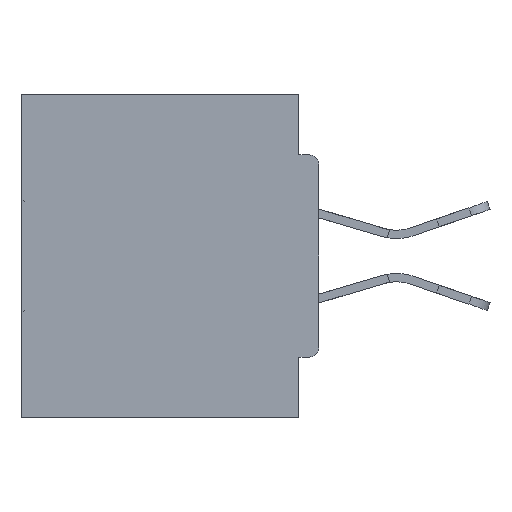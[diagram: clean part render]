
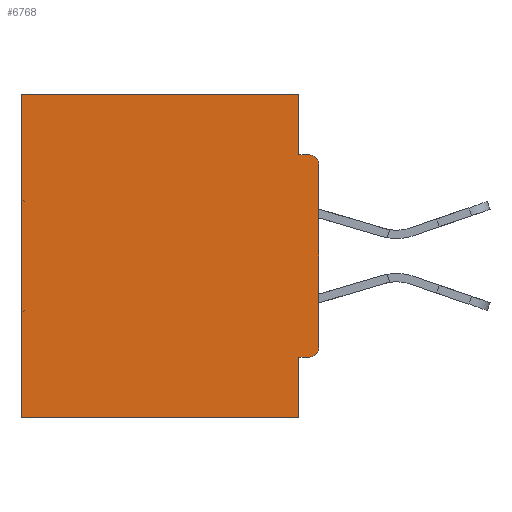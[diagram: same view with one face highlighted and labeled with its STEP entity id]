
A CAD part, left-side view. The second image highlights one B-rep face of the part: STEP entity #6768.
In plain terms, the highlighted planar face has unit normal (-1, 0, 0).
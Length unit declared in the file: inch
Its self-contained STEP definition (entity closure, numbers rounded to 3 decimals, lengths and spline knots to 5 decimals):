
#62 = ORIENTED_EDGE ( 'NONE', *, *, #31509, .F. ) ;
#794 = VERTEX_POINT ( 'NONE', #36047 ) ;
#926 = VECTOR ( 'NONE', #1300, 39.37008 ) ;
#1300 = DIRECTION ( 'NONE',  ( 0., 1., 0. ) ) ;
#1567 = CARTESIAN_POINT ( 'NONE',  ( 0.298, 0.031, 0. ) ) ;
#2746 = CARTESIAN_POINT ( 'NONE',  ( 0.298, 0., -0.4065 ) ) ;
#2751 = ORIENTED_EDGE ( 'NONE', *, *, #35384, .F. ) ;
#5002 = VECTOR ( 'NONE', #16791, 39.37008 ) ;
#5671 = EDGE_CURVE ( 'NONE', #35676, #30336, #21587, .T. ) ;
#5812 = EDGE_CURVE ( 'NONE', #794, #27218, #32672, .T. ) ;
#5937 = ORIENTED_EDGE ( 'NONE', *, *, #7965, .F. ) ;
#6116 = CARTESIAN_POINT ( 'NONE',  ( 0.298, 0.46, 0. ) ) ;
#6743 = DIRECTION ( 'NONE',  ( 0., 0., -1. ) ) ;
#6768 = ADVANCED_FACE ( 'NONE', ( #29023 ), #19098, .F. ) ;
#7354 = CARTESIAN_POINT ( 'NONE',  ( 0.298, 0.46, 0. ) ) ;
#7462 = EDGE_CURVE ( 'NONE', #38261, #15851, #22695, .T. ) ;
#7965 = EDGE_CURVE ( 'NONE', #15851, #39488, #16873, .T. ) ;
#7985 = EDGE_CURVE ( 'NONE', #38261, #21097, #32724, .T. ) ;
#8307 = CARTESIAN_POINT ( 'NONE',  ( 0.298, 0., 0. ) ) ;
#8450 = AXIS2_PLACEMENT_3D ( 'NONE', #27427, #27571, #27730 ) ;
#8752 = ORIENTED_EDGE ( 'NONE', *, *, #7462, .F. ) ;
#8756 = ORIENTED_EDGE ( 'NONE', *, *, #10908, .T. ) ;
#8794 = VECTOR ( 'NONE', #23334, 39.37008 ) ;
#9895 = CARTESIAN_POINT ( 'NONE',  ( 0.298, 0., -0.5 ) ) ;
#10908 = EDGE_CURVE ( 'NONE', #33389, #27218, #39284, .T. ) ;
#10940 = CARTESIAN_POINT ( 'NONE',  ( 0.298, 0.015, -0.4065 ) ) ;
#11133 = CARTESIAN_POINT ( 'NONE',  ( 0.298, 0., 0. ) ) ;
#11499 = ORIENTED_EDGE ( 'NONE', *, *, #35125, .F. ) ;
#12402 = DIRECTION ( 'NONE',  ( 0., -1., 0. ) ) ;
#13107 = CARTESIAN_POINT ( 'NONE',  ( 0.298, 0., -0.3915 ) ) ;
#13188 = DIRECTION ( 'NONE',  ( 0., 1., 0. ) ) ;
#14216 = CARTESIAN_POINT ( 'NONE',  ( 0.298, 0.015, -0.3915 ) ) ;
#15851 = VERTEX_POINT ( 'NONE', #24425 ) ;
#16791 = DIRECTION ( 'NONE',  ( 0., 0., -1. ) ) ;
#16873 = LINE ( 'NONE', #17031, #41701 ) ;
#17031 = CARTESIAN_POINT ( 'NONE',  ( 0.298, 0.031, -0.5 ) ) ;
#18262 = DIRECTION ( 'NONE',  ( 0., 1., 0. ) ) ;
#18898 = VECTOR ( 'NONE', #12402, 39.37008 ) ;
#19098 = PLANE ( 'NONE',  #39483 ) ;
#19381 = CARTESIAN_POINT ( 'NONE',  ( 0.298, 0., 0. ) ) ;
#20803 = ORIENTED_EDGE ( 'NONE', *, *, #5671, .T. ) ;
#21097 = VERTEX_POINT ( 'NONE', #13107 ) ;
#21587 = LINE ( 'NONE', #6116, #8794 ) ;
#22084 = EDGE_CURVE ( 'NONE', #43184, #35676, #33359, .T. ) ;
#22695 = LINE ( 'NONE', #2746, #29596 ) ;
#23334 = DIRECTION ( 'NONE',  ( 0., 0., -1. ) ) ;
#23855 = CARTESIAN_POINT ( 'NONE',  ( 0.298, 0.031, -0.5 ) ) ;
#24382 = LINE ( 'NONE', #11133, #39679 ) ;
#24425 = CARTESIAN_POINT ( 'NONE',  ( 0.298, 0.031, -0.4065 ) ) ;
#25900 = ORIENTED_EDGE ( 'NONE', *, *, #7985, .T. ) ;
#26260 = EDGE_LOOP ( 'NONE', ( #8756, #35823, #62, #38608, #20803, #2751, #5937, #8752, #25900, #11499 ) ) ;
#26983 = VECTOR ( 'NONE', #13188, 39.37008 ) ;
#27023 = DIRECTION ( 'NONE',  ( -1., 0., 0. ) ) ;
#27218 = VERTEX_POINT ( 'NONE', #32149 ) ;
#27427 = CARTESIAN_POINT ( 'NONE',  ( 0.298, 0.015, -0.1085 ) ) ;
#27571 = DIRECTION ( 'NONE',  ( -1., 0., 0. ) ) ;
#27697 = DIRECTION ( 'NONE',  ( 0., 0., -1. ) ) ;
#27730 = DIRECTION ( 'NONE',  ( 0., 0., -1. ) ) ;
#29023 = FACE_OUTER_BOUND ( 'NONE', #26260, .T. ) ;
#29252 = CARTESIAN_POINT ( 'NONE',  ( 0.298, 0., -0.0935 ) ) ;
#29596 = VECTOR ( 'NONE', #18262, 39.37008 ) ;
#30129 = CARTESIAN_POINT ( 'NONE',  ( 0.298, 0.46, -0.5 ) ) ;
#30336 = VERTEX_POINT ( 'NONE', #30129 ) ;
#31509 = EDGE_CURVE ( 'NONE', #43184, #794, #40510, .T. ) ;
#32149 = CARTESIAN_POINT ( 'NONE',  ( 0.298, 0.015, -0.0935 ) ) ;
#32672 = LINE ( 'NONE', #29252, #18898 ) ;
#32724 = CIRCLE ( 'NONE', #40408, 0.015 ) ;
#33359 = LINE ( 'NONE', #8307, #926 ) ;
#33389 = VERTEX_POINT ( 'NONE', #33684 ) ;
#33684 = CARTESIAN_POINT ( 'NONE',  ( 0.298, 0., -0.1085 ) ) ;
#35125 = EDGE_CURVE ( 'NONE', #33389, #21097, #24382, .T. ) ;
#35384 = EDGE_CURVE ( 'NONE', #39488, #30336, #36001, .T. ) ;
#35676 = VERTEX_POINT ( 'NONE', #7354 ) ;
#35823 = ORIENTED_EDGE ( 'NONE', *, *, #5812, .F. ) ;
#36001 = LINE ( 'NONE', #9895, #26983 ) ;
#36047 = CARTESIAN_POINT ( 'NONE',  ( 0.298, 0.031, -0.0935 ) ) ;
#38261 = VERTEX_POINT ( 'NONE', #10940 ) ;
#38608 = ORIENTED_EDGE ( 'NONE', *, *, #22084, .T. ) ;
#39284 = CIRCLE ( 'NONE', #8450, 0.015 ) ;
#39483 = AXIS2_PLACEMENT_3D ( 'NONE', #19381, #40666, #43477 ) ;
#39488 = VERTEX_POINT ( 'NONE', #43769 ) ;
#39679 = VECTOR ( 'NONE', #27697, 39.37008 ) ;
#40408 = AXIS2_PLACEMENT_3D ( 'NONE', #14216, #27023, #6743 ) ;
#40510 = LINE ( 'NONE', #23855, #5002 ) ;
#40666 = DIRECTION ( 'NONE',  ( 1., 0., 0. ) ) ;
#40794 = DIRECTION ( 'NONE',  ( 0., 0., -1. ) ) ;
#41701 = VECTOR ( 'NONE', #40794, 39.37008 ) ;
#43184 = VERTEX_POINT ( 'NONE', #1567 ) ;
#43477 = DIRECTION ( 'NONE',  ( 0., 0., -1. ) ) ;
#43769 = CARTESIAN_POINT ( 'NONE',  ( 0.298, 0.031, -0.5 ) ) ;
